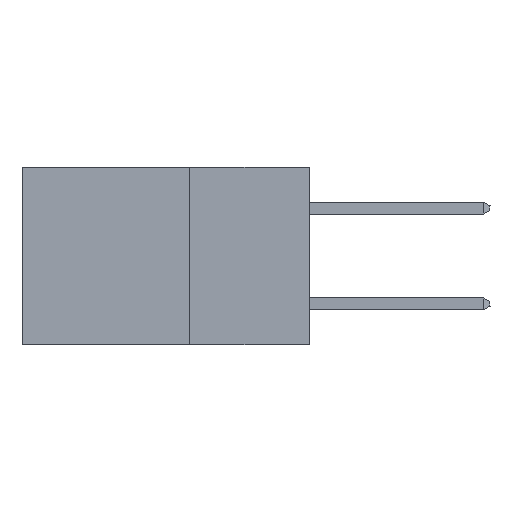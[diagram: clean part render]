
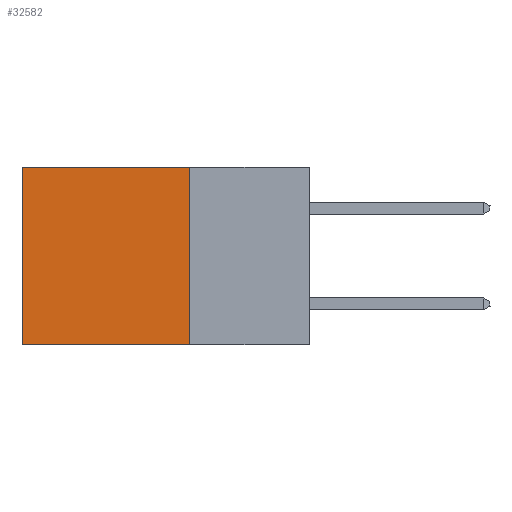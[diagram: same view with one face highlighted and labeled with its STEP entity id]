
A CAD part, left-side view. The second image highlights one B-rep face of the part: STEP entity #32582.
In plain terms, the highlighted planar face has unit normal (-1, 0, 0).
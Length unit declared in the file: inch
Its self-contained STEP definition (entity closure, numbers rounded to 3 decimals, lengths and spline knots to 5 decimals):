
#213 = LINE ( 'NONE', #17364, #4887 ) ;
#280 = CARTESIAN_POINT ( 'NONE',  ( 0.2875, 0.25, 0. ) ) ;
#1134 = VECTOR ( 'NONE', #17678, 39.37008 ) ;
#4608 = ORIENTED_EDGE ( 'NONE', *, *, #34662, .F. ) ;
#4887 = VECTOR ( 'NONE', #29287, 39.37008 ) ;
#5518 = EDGE_CURVE ( 'NONE', #13795, #32717, #24261, .T. ) ;
#6020 = ORIENTED_EDGE ( 'NONE', *, *, #30926, .T. ) ;
#6920 = CARTESIAN_POINT ( 'NONE',  ( 0.2875, 0.25, 0. ) ) ;
#10958 = AXIS2_PLACEMENT_3D ( 'NONE', #280, #21279, #24414 ) ;
#12555 = DIRECTION ( 'NONE',  ( 0., 0., -1. ) ) ;
#13795 = VERTEX_POINT ( 'NONE', #16034 ) ;
#15898 = CARTESIAN_POINT ( 'NONE',  ( 0.2875, 0.25, -0.37 ) ) ;
#15987 = CARTESIAN_POINT ( 'NONE',  ( 0.2875, 0.6, -0.37 ) ) ;
#16034 = CARTESIAN_POINT ( 'NONE',  ( 0.2875, 0.25, 0. ) ) ;
#16110 = EDGE_CURVE ( 'NONE', #27004, #18928, #30241, .T. ) ;
#16298 = VECTOR ( 'NONE', #12555, 39.37008 ) ;
#17268 = FACE_OUTER_BOUND ( 'NONE', #38675, .T. ) ;
#17364 = CARTESIAN_POINT ( 'NONE',  ( 0.2875, 0.25, -0.37 ) ) ;
#17678 = DIRECTION ( 'NONE',  ( 0., 0., -1. ) ) ;
#18928 = VERTEX_POINT ( 'NONE', #15987 ) ;
#21279 = DIRECTION ( 'NONE',  ( 1., 0., 0. ) ) ;
#21494 = ORIENTED_EDGE ( 'NONE', *, *, #16110, .T. ) ;
#22054 = LINE ( 'NONE', #31534, #34743 ) ;
#24261 = LINE ( 'NONE', #6920, #16298 ) ;
#24414 = DIRECTION ( 'NONE',  ( 0., 0., -1. ) ) ;
#24541 = ORIENTED_EDGE ( 'NONE', *, *, #5518, .F. ) ;
#25357 = DIRECTION ( 'NONE',  ( 0., 1., 0. ) ) ;
#26707 = CARTESIAN_POINT ( 'NONE',  ( 0.2875, 0.6, 0. ) ) ;
#27004 = VERTEX_POINT ( 'NONE', #26707 ) ;
#29287 = DIRECTION ( 'NONE',  ( 0., 1., 0. ) ) ;
#30241 = LINE ( 'NONE', #32247, #1134 ) ;
#30926 = EDGE_CURVE ( 'NONE', #13795, #27004, #22054, .T. ) ;
#31534 = CARTESIAN_POINT ( 'NONE',  ( 0.2875, 0.25, 0. ) ) ;
#32247 = CARTESIAN_POINT ( 'NONE',  ( 0.2875, 0.6, 0. ) ) ;
#32582 = ADVANCED_FACE ( 'NONE', ( #17268 ), #36217, .F. ) ;
#32717 = VERTEX_POINT ( 'NONE', #15898 ) ;
#34662 = EDGE_CURVE ( 'NONE', #32717, #18928, #213, .T. ) ;
#34743 = VECTOR ( 'NONE', #25357, 39.37008 ) ;
#36217 = PLANE ( 'NONE',  #10958 ) ;
#38675 = EDGE_LOOP ( 'NONE', ( #21494, #4608, #24541, #6020 ) ) ;
